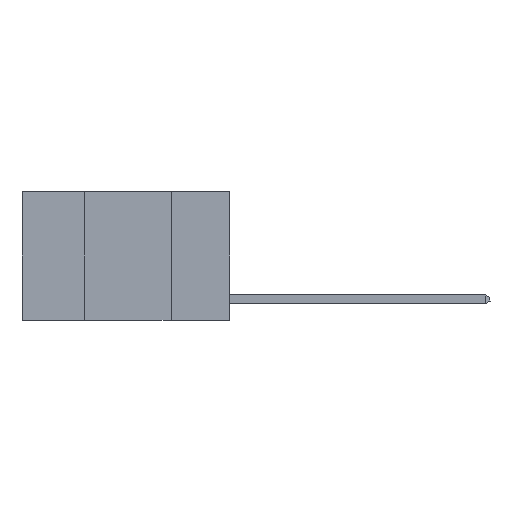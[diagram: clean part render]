
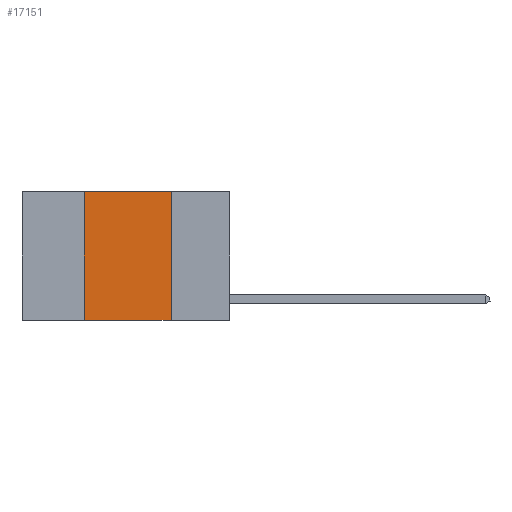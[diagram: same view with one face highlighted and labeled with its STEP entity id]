
A CAD part, left-side view. The second image highlights one B-rep face of the part: STEP entity #17151.
In plain terms, the highlighted planar face has unit normal (-1, 0, 0).
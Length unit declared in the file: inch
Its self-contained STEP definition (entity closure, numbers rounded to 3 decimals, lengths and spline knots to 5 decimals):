
#346 = VERTEX_POINT ( 'NONE', #26777 ) ;
#535 = DIRECTION ( 'NONE',  ( 1., 0., 0. ) ) ;
#656 = ORIENTED_EDGE ( 'NONE', *, *, #9015, .F. ) ;
#1064 = LINE ( 'NONE', #3179, #6963 ) ;
#1239 = CARTESIAN_POINT ( 'NONE',  ( 0., 0.17, -0.37 ) ) ;
#3179 = CARTESIAN_POINT ( 'NONE',  ( 0., 0.42, 0. ) ) ;
#3643 = LINE ( 'NONE', #24836, #9516 ) ;
#5514 = CARTESIAN_POINT ( 'NONE',  ( 0., 0.17, 0. ) ) ;
#6963 = VECTOR ( 'NONE', #20310, 39.37008 ) ;
#8518 = LINE ( 'NONE', #5514, #14330 ) ;
#9015 = EDGE_CURVE ( 'NONE', #11349, #28108, #8518, .T. ) ;
#9054 = EDGE_CURVE ( 'NONE', #346, #28335, #1064, .T. ) ;
#9356 = DIRECTION ( 'NONE',  ( 0., -1., 0. ) ) ;
#9516 = VECTOR ( 'NONE', #10537, 39.37008 ) ;
#10537 = DIRECTION ( 'NONE',  ( 0., -1., 0. ) ) ;
#10933 = FACE_OUTER_BOUND ( 'NONE', #14124, .T. ) ;
#11349 = VERTEX_POINT ( 'NONE', #16792 ) ;
#13952 = EDGE_CURVE ( 'NONE', #346, #28108, #3643, .T. ) ;
#14124 = EDGE_LOOP ( 'NONE', ( #656, #29462, #29103, #23217 ) ) ;
#14330 = VECTOR ( 'NONE', #22490, 39.37008 ) ;
#15434 = PLANE ( 'NONE',  #27023 ) ;
#16792 = CARTESIAN_POINT ( 'NONE',  ( 0., 0.17, 0. ) ) ;
#17151 = ADVANCED_FACE ( 'NONE', ( #10933 ), #15434, .F. ) ;
#17705 = CARTESIAN_POINT ( 'NONE',  ( 0., 0.6, 0. ) ) ;
#17797 = DIRECTION ( 'NONE',  ( 0., 0., -1. ) ) ;
#20310 = DIRECTION ( 'NONE',  ( 0., 0., 1. ) ) ;
#21376 = CARTESIAN_POINT ( 'NONE',  ( 0., 0.6, 0. ) ) ;
#22490 = DIRECTION ( 'NONE',  ( 0., 0., -1. ) ) ;
#23079 = EDGE_CURVE ( 'NONE', #28335, #11349, #24230, .T. ) ;
#23217 = ORIENTED_EDGE ( 'NONE', *, *, #13952, .T. ) ;
#23730 = CARTESIAN_POINT ( 'NONE',  ( 0., 0.42, 0. ) ) ;
#24230 = LINE ( 'NONE', #21376, #29698 ) ;
#24836 = CARTESIAN_POINT ( 'NONE',  ( 0., 0.6, -0.37 ) ) ;
#26777 = CARTESIAN_POINT ( 'NONE',  ( 0., 0.42, -0.37 ) ) ;
#27023 = AXIS2_PLACEMENT_3D ( 'NONE', #17705, #535, #17797 ) ;
#28108 = VERTEX_POINT ( 'NONE', #1239 ) ;
#28335 = VERTEX_POINT ( 'NONE', #23730 ) ;
#29103 = ORIENTED_EDGE ( 'NONE', *, *, #9054, .F. ) ;
#29462 = ORIENTED_EDGE ( 'NONE', *, *, #23079, .F. ) ;
#29698 = VECTOR ( 'NONE', #9356, 39.37008 ) ;
